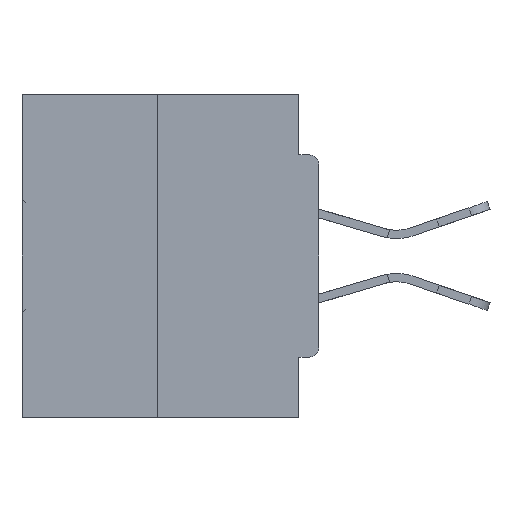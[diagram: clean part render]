
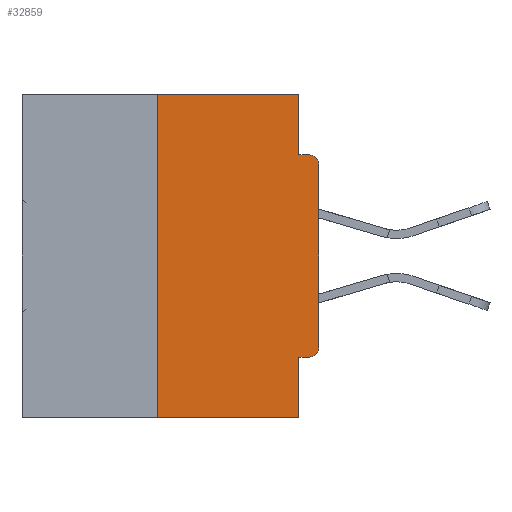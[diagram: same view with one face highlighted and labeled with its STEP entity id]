
A CAD part, left-side view. The second image highlights one B-rep face of the part: STEP entity #32859.
In plain terms, the highlighted planar face has unit normal (-1, 0, 0).
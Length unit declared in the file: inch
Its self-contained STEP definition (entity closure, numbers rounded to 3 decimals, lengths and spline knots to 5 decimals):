
#612 = LINE ( 'NONE', #13921, #22856 ) ;
#955 = VERTEX_POINT ( 'NONE', #19464 ) ;
#1159 = DIRECTION ( 'NONE',  ( 0., 0., 1. ) ) ;
#1776 = VECTOR ( 'NONE', #1159, 39.37008 ) ;
#2392 = LINE ( 'NONE', #43462, #4122 ) ;
#2395 = ORIENTED_EDGE ( 'NONE', *, *, #18389, .T. ) ;
#3592 = ORIENTED_EDGE ( 'NONE', *, *, #15384, .T. ) ;
#3895 = EDGE_CURVE ( 'NONE', #38779, #39372, #10032, .T. ) ;
#4122 = VECTOR ( 'NONE', #40547, 39.37008 ) ;
#5657 = DIRECTION ( 'NONE',  ( -1., 0., 0. ) ) ;
#5676 = VECTOR ( 'NONE', #7632, 39.37008 ) ;
#6424 = LINE ( 'NONE', #33985, #21796 ) ;
#6595 = VECTOR ( 'NONE', #42197, 39.37008 ) ;
#6689 = VERTEX_POINT ( 'NONE', #34910 ) ;
#6927 = DIRECTION ( 'NONE',  ( 1., 0., 0. ) ) ;
#7593 = DIRECTION ( 'NONE',  ( 0., 1., 0. ) ) ;
#7632 = DIRECTION ( 'NONE',  ( 0., 0., 1. ) ) ;
#8084 = CARTESIAN_POINT ( 'NONE',  ( 0., 0.031, -0.5 ) ) ;
#10032 = LINE ( 'NONE', #22910, #27564 ) ;
#11117 = ORIENTED_EDGE ( 'NONE', *, *, #25471, .T. ) ;
#12188 = ORIENTED_EDGE ( 'NONE', *, *, #37225, .T. ) ;
#12419 = CARTESIAN_POINT ( 'NONE',  ( 0., 0.015, -0.1085 ) ) ;
#12580 = CARTESIAN_POINT ( 'NONE',  ( 0., 0.031, 0. ) ) ;
#13548 = AXIS2_PLACEMENT_3D ( 'NONE', #12419, #5657, #43580 ) ;
#13921 = CARTESIAN_POINT ( 'NONE',  ( 0., 0., -0.4065 ) ) ;
#14199 = VERTEX_POINT ( 'NONE', #21839 ) ;
#15384 = EDGE_CURVE ( 'NONE', #6689, #955, #28435, .T. ) ;
#15485 = VERTEX_POINT ( 'NONE', #41520 ) ;
#16251 = ORIENTED_EDGE ( 'NONE', *, *, #37752, .F. ) ;
#17090 = PLANE ( 'NONE',  #26099 ) ;
#18086 = CARTESIAN_POINT ( 'NONE',  ( 0., 0.25, 0. ) ) ;
#18389 = EDGE_CURVE ( 'NONE', #19714, #33944, #41686, .T. ) ;
#19464 = CARTESIAN_POINT ( 'NONE',  ( 0., 0., -0.1085 ) ) ;
#19714 = VERTEX_POINT ( 'NONE', #27705 ) ;
#20480 = DIRECTION ( 'NONE',  ( 0., 0., -1. ) ) ;
#20696 = CARTESIAN_POINT ( 'NONE',  ( 0., 0.46, 0. ) ) ;
#20949 = ORIENTED_EDGE ( 'NONE', *, *, #29510, .F. ) ;
#21796 = VECTOR ( 'NONE', #31042, 39.37008 ) ;
#21839 = CARTESIAN_POINT ( 'NONE',  ( 0., 0.015, -0.4065 ) ) ;
#22064 = VERTEX_POINT ( 'NONE', #33848 ) ;
#22856 = VECTOR ( 'NONE', #7593, 39.37008 ) ;
#22910 = CARTESIAN_POINT ( 'NONE',  ( 0., 0.031, 0. ) ) ;
#24139 = CIRCLE ( 'NONE', #28192, 0.015 ) ;
#25471 = EDGE_CURVE ( 'NONE', #955, #22064, #39536, .T. ) ;
#26099 = AXIS2_PLACEMENT_3D ( 'NONE', #20696, #6927, #20480 ) ;
#27411 = CARTESIAN_POINT ( 'NONE',  ( 0., 0.25, 0. ) ) ;
#27564 = VECTOR ( 'NONE', #36688, 39.37008 ) ;
#27705 = CARTESIAN_POINT ( 'NONE',  ( 0., 0.25, -0.5 ) ) ;
#27903 = CARTESIAN_POINT ( 'NONE',  ( 0., 0.031, -0.0935 ) ) ;
#28192 = AXIS2_PLACEMENT_3D ( 'NONE', #30270, #34318, #33427 ) ;
#28435 = LINE ( 'NONE', #38591, #5676 ) ;
#28535 = EDGE_CURVE ( 'NONE', #15485, #33944, #39034, .T. ) ;
#28600 = CARTESIAN_POINT ( 'NONE',  ( 0., 0.46, -0.5 ) ) ;
#29302 = ORIENTED_EDGE ( 'NONE', *, *, #36898, .F. ) ;
#29510 = EDGE_CURVE ( 'NONE', #39372, #22064, #6424, .T. ) ;
#29686 = EDGE_LOOP ( 'NONE', ( #36638, #29302, #2395, #43314, #16251, #12188, #3592, #11117, #20949, #35763 ) ) ;
#30270 = CARTESIAN_POINT ( 'NONE',  ( 0., 0.015, -0.3915 ) ) ;
#31042 = DIRECTION ( 'NONE',  ( 0., -1., 0. ) ) ;
#32859 = ADVANCED_FACE ( 'NONE', ( #37427 ), #17090, .F. ) ;
#33427 = DIRECTION ( 'NONE',  ( 0., 0., -1. ) ) ;
#33848 = CARTESIAN_POINT ( 'NONE',  ( 0., 0.015, -0.0935 ) ) ;
#33944 = VERTEX_POINT ( 'NONE', #43524 ) ;
#33985 = CARTESIAN_POINT ( 'NONE',  ( 0., 0., -0.0935 ) ) ;
#34318 = DIRECTION ( 'NONE',  ( -1., 0., 0. ) ) ;
#34910 = CARTESIAN_POINT ( 'NONE',  ( 0., 0., -0.3915 ) ) ;
#35476 = LINE ( 'NONE', #18086, #1776 ) ;
#35763 = ORIENTED_EDGE ( 'NONE', *, *, #3895, .F. ) ;
#36638 = ORIENTED_EDGE ( 'NONE', *, *, #38021, .F. ) ;
#36688 = DIRECTION ( 'NONE',  ( 0., 0., -1. ) ) ;
#36898 = EDGE_CURVE ( 'NONE', #19714, #40693, #35476, .T. ) ;
#37225 = EDGE_CURVE ( 'NONE', #14199, #6689, #24139, .T. ) ;
#37427 = FACE_OUTER_BOUND ( 'NONE', #29686, .T. ) ;
#37752 = EDGE_CURVE ( 'NONE', #14199, #15485, #612, .T. ) ;
#38021 = EDGE_CURVE ( 'NONE', #40693, #38779, #2392, .T. ) ;
#38591 = CARTESIAN_POINT ( 'NONE',  ( 0., 0., 0. ) ) ;
#38779 = VERTEX_POINT ( 'NONE', #12580 ) ;
#39034 = LINE ( 'NONE', #8084, #6595 ) ;
#39372 = VERTEX_POINT ( 'NONE', #27903 ) ;
#39536 = CIRCLE ( 'NONE', #13548, 0.015 ) ;
#39659 = VECTOR ( 'NONE', #42349, 39.37008 ) ;
#40547 = DIRECTION ( 'NONE',  ( 0., -1., 0. ) ) ;
#40693 = VERTEX_POINT ( 'NONE', #27411 ) ;
#41520 = CARTESIAN_POINT ( 'NONE',  ( 0., 0.031, -0.4065 ) ) ;
#41686 = LINE ( 'NONE', #28600, #39659 ) ;
#42197 = DIRECTION ( 'NONE',  ( 0., 0., -1. ) ) ;
#42349 = DIRECTION ( 'NONE',  ( 0., -1., 0. ) ) ;
#43314 = ORIENTED_EDGE ( 'NONE', *, *, #28535, .F. ) ;
#43462 = CARTESIAN_POINT ( 'NONE',  ( 0., 0.46, 0. ) ) ;
#43524 = CARTESIAN_POINT ( 'NONE',  ( 0., 0.031, -0.5 ) ) ;
#43580 = DIRECTION ( 'NONE',  ( 0., 0., -1. ) ) ;
